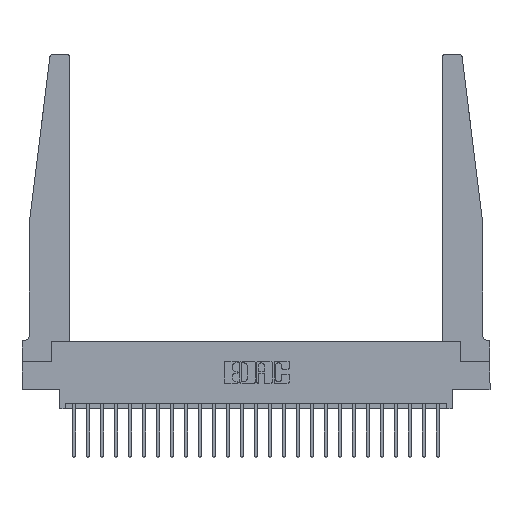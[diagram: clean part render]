
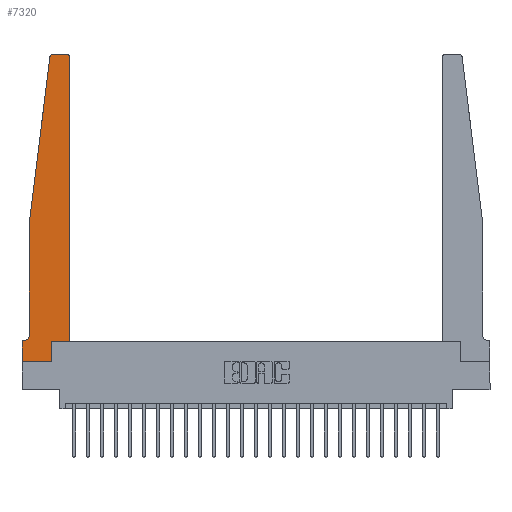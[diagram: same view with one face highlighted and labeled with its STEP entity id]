
A CAD part, top view. The second image highlights one B-rep face of the part: STEP entity #7320.
In plain terms, the highlighted planar face has unit normal (0, 0, 1).
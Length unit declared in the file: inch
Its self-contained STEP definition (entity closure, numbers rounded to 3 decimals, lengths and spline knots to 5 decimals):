
#179 = DIRECTION ( 'NONE',  ( 0., 1., 0. ) ) ;
#450 = DIRECTION ( 'NONE',  ( 0., 0., 1. ) ) ;
#580 = VERTEX_POINT ( 'NONE', #13751 ) ;
#949 = DIRECTION ( 'NONE',  ( 1., 0., 0. ) ) ;
#1013 = CARTESIAN_POINT ( 'NONE',  ( 0.425, 2.72, 0.37 ) ) ;
#1115 = DIRECTION ( 'NONE',  ( -0.122, -0.992, 0. ) ) ;
#1154 = CARTESIAN_POINT ( 'NONE',  ( 0.065, 1.25, 0.37 ) ) ;
#1348 = CARTESIAN_POINT ( 'NONE',  ( 0., 0.1875, 0.37 ) ) ;
#1594 = EDGE_CURVE ( 'NONE', #24060, #5919, #8456, .T. ) ;
#1705 = EDGE_CURVE ( 'NONE', #1788, #580, #6138, .T. ) ;
#1740 = VECTOR ( 'NONE', #6687, 39.37008 ) ;
#1788 = VERTEX_POINT ( 'NONE', #7067 ) ;
#1837 = CARTESIAN_POINT ( 'NONE',  ( 0.425, 0.18, 0.37 ) ) ;
#2057 = LINE ( 'NONE', #2178, #12835 ) ;
#2178 = CARTESIAN_POINT ( 'NONE',  ( 0., 0., 0.37 ) ) ;
#2996 = DIRECTION ( 'NONE',  ( -1., 0., 0. ) ) ;
#2999 = CARTESIAN_POINT ( 'NONE',  ( 0.065, 1.25, 0.37 ) ) ;
#3162 = EDGE_CURVE ( 'NONE', #580, #24060, #5437, .T. ) ;
#3292 = CARTESIAN_POINT ( 'NONE',  ( 0.065, 0.1875, 0.37 ) ) ;
#4024 = EDGE_CURVE ( 'NONE', #19753, #20650, #20325, .T. ) ;
#4641 = LINE ( 'NONE', #10240, #13375 ) ;
#4649 = EDGE_LOOP ( 'NONE', ( #15118, #6435, #18858, #8255, #20187, #4933, #20471, #10739, #12929, #7818, #15611, #16040 ) ) ;
#4894 = DIRECTION ( 'NONE',  ( 0., 0., -1. ) ) ;
#4933 = ORIENTED_EDGE ( 'NONE', *, *, #3162, .T. ) ;
#5437 = LINE ( 'NONE', #3292, #19660 ) ;
#5580 = FACE_OUTER_BOUND ( 'NONE', #4649, .T. ) ;
#5904 = CIRCLE ( 'NONE', #11184, 0.03 ) ;
#5919 = VERTEX_POINT ( 'NONE', #9041 ) ;
#6138 = CIRCLE ( 'NONE', #10612, 0.05 ) ;
#6435 = ORIENTED_EDGE ( 'NONE', *, *, #24457, .T. ) ;
#6673 = VERTEX_POINT ( 'NONE', #24251 ) ;
#6687 = DIRECTION ( 'NONE',  ( 0., -1., 0. ) ) ;
#6768 = EDGE_CURVE ( 'NONE', #18571, #15068, #19288, .T. ) ;
#7067 = CARTESIAN_POINT ( 'NONE',  ( 0.065, 0.2375, 0.37 ) ) ;
#7094 = VECTOR ( 'NONE', #8887, 39.37008 ) ;
#7268 = VERTEX_POINT ( 'NONE', #7389 ) ;
#7320 = ADVANCED_FACE ( 'NONE', ( #5580 ), #15097, .T. ) ;
#7389 = CARTESIAN_POINT ( 'NONE',  ( 0.2605, 0., 0.37 ) ) ;
#7818 = ORIENTED_EDGE ( 'NONE', *, *, #8459, .T. ) ;
#7862 = CARTESIAN_POINT ( 'NONE',  ( 0.24675, 2.72367, 0.37 ) ) ;
#8255 = ORIENTED_EDGE ( 'NONE', *, *, #20680, .T. ) ;
#8456 = LINE ( 'NONE', #13900, #1740 ) ;
#8459 = EDGE_CURVE ( 'NONE', #18485, #18571, #16878, .T. ) ;
#8887 = DIRECTION ( 'NONE',  ( 0., -1., 0. ) ) ;
#9041 = CARTESIAN_POINT ( 'NONE',  ( 0., 0., 0.37 ) ) ;
#10240 = CARTESIAN_POINT ( 'NONE',  ( 0.25, 2.75, 0.37 ) ) ;
#10612 = AXIS2_PLACEMENT_3D ( 'NONE', #24394, #4894, #10750 ) ;
#10666 = VECTOR ( 'NONE', #23857, 39.37008 ) ;
#10739 = ORIENTED_EDGE ( 'NONE', *, *, #24734, .T. ) ;
#10750 = DIRECTION ( 'NONE',  ( -1., 0., 0. ) ) ;
#10883 = EDGE_CURVE ( 'NONE', #6673, #17629, #4641, .T. ) ;
#10956 = DIRECTION ( 'NONE',  ( 0., 0., 1. ) ) ;
#11184 = AXIS2_PLACEMENT_3D ( 'NONE', #20273, #10956, #24223 ) ;
#11426 = EDGE_CURVE ( 'NONE', #15068, #6673, #12163, .T. ) ;
#11549 = DIRECTION ( 'NONE',  ( 0., 0., 1. ) ) ;
#12163 = CIRCLE ( 'NONE', #17413, 0.03 ) ;
#12815 = CARTESIAN_POINT ( 'NONE',  ( 0.2605, 0.18, 0.37 ) ) ;
#12820 = VECTOR ( 'NONE', #15235, 39.37008 ) ;
#12835 = VECTOR ( 'NONE', #15844, 39.37008 ) ;
#12929 = ORIENTED_EDGE ( 'NONE', *, *, #13862, .T. ) ;
#13077 = CARTESIAN_POINT ( 'NONE',  ( 0., 0.1875, 0.37 ) ) ;
#13175 = CARTESIAN_POINT ( 'NONE',  ( 0.065, 1.25, 0.37 ) ) ;
#13375 = VECTOR ( 'NONE', #2996, 39.37008 ) ;
#13462 = CARTESIAN_POINT ( 'NONE',  ( 0.425, 0.18, 0.37 ) ) ;
#13751 = CARTESIAN_POINT ( 'NONE',  ( 0.015, 0.1875, 0.37 ) ) ;
#13862 = EDGE_CURVE ( 'NONE', #7268, #18485, #19541, .T. ) ;
#13900 = CARTESIAN_POINT ( 'NONE',  ( 0., 0., 0.37 ) ) ;
#14173 = CARTESIAN_POINT ( 'NONE',  ( 0.425, 0.18, 0.37 ) ) ;
#14923 = CARTESIAN_POINT ( 'NONE',  ( 0.27653, 2.75, 0.37 ) ) ;
#15068 = VERTEX_POINT ( 'NONE', #1013 ) ;
#15097 = PLANE ( 'NONE',  #16312 ) ;
#15118 = ORIENTED_EDGE ( 'NONE', *, *, #10883, .T. ) ;
#15235 = DIRECTION ( 'NONE',  ( 1., 0., 0. ) ) ;
#15611 = ORIENTED_EDGE ( 'NONE', *, *, #6768, .T. ) ;
#15844 = DIRECTION ( 'NONE',  ( 1., 0., 0. ) ) ;
#16040 = ORIENTED_EDGE ( 'NONE', *, *, #11426, .T. ) ;
#16127 = CARTESIAN_POINT ( 'NONE',  ( 0.2605, 0.18, 0.37 ) ) ;
#16312 = AXIS2_PLACEMENT_3D ( 'NONE', #13077, #11549, #20760 ) ;
#16878 = LINE ( 'NONE', #13462, #12820 ) ;
#17413 = AXIS2_PLACEMENT_3D ( 'NONE', #17906, #450, #949 ) ;
#17629 = VERTEX_POINT ( 'NONE', #14923 ) ;
#17906 = CARTESIAN_POINT ( 'NONE',  ( 0.395, 2.72, 0.37 ) ) ;
#18485 = VERTEX_POINT ( 'NONE', #12815 ) ;
#18571 = VERTEX_POINT ( 'NONE', #14173 ) ;
#18740 = DIRECTION ( 'NONE',  ( -1., 0., 0. ) ) ;
#18821 = VECTOR ( 'NONE', #179, 39.37008 ) ;
#18858 = ORIENTED_EDGE ( 'NONE', *, *, #4024, .T. ) ;
#19288 = LINE ( 'NONE', #1837, #18821 ) ;
#19541 = LINE ( 'NONE', #16127, #10666 ) ;
#19660 = VECTOR ( 'NONE', #18740, 39.37008 ) ;
#19753 = VERTEX_POINT ( 'NONE', #7862 ) ;
#20187 = ORIENTED_EDGE ( 'NONE', *, *, #1705, .T. ) ;
#20273 = CARTESIAN_POINT ( 'NONE',  ( 0.27653, 2.72, 0.37 ) ) ;
#20325 = LINE ( 'NONE', #2999, #24757 ) ;
#20365 = LINE ( 'NONE', #13175, #7094 ) ;
#20471 = ORIENTED_EDGE ( 'NONE', *, *, #1594, .T. ) ;
#20650 = VERTEX_POINT ( 'NONE', #1154 ) ;
#20680 = EDGE_CURVE ( 'NONE', #20650, #1788, #20365, .T. ) ;
#20760 = DIRECTION ( 'NONE',  ( 1., 0., 0. ) ) ;
#23857 = DIRECTION ( 'NONE',  ( 0., 1., 0. ) ) ;
#24060 = VERTEX_POINT ( 'NONE', #1348 ) ;
#24223 = DIRECTION ( 'NONE',  ( 1., 0., 0. ) ) ;
#24251 = CARTESIAN_POINT ( 'NONE',  ( 0.395, 2.75, 0.37 ) ) ;
#24394 = CARTESIAN_POINT ( 'NONE',  ( 0.015, 0.2375, 0.37 ) ) ;
#24457 = EDGE_CURVE ( 'NONE', #17629, #19753, #5904, .T. ) ;
#24734 = EDGE_CURVE ( 'NONE', #5919, #7268, #2057, .T. ) ;
#24757 = VECTOR ( 'NONE', #1115, 39.37008 ) ;
